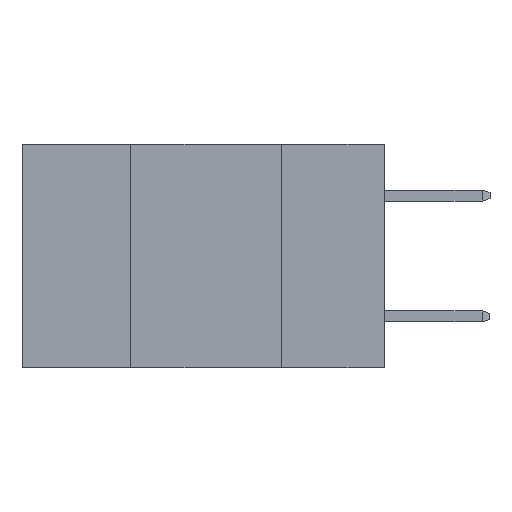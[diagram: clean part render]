
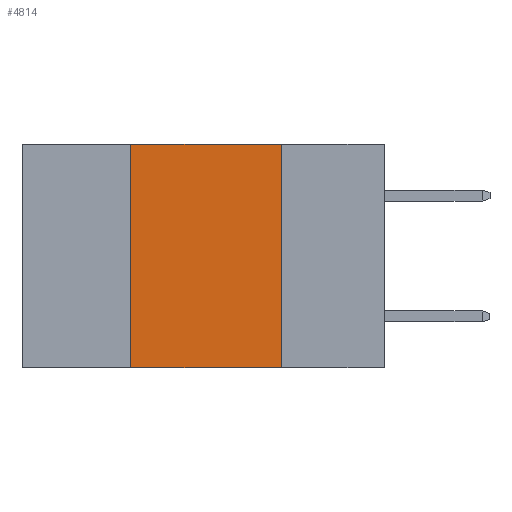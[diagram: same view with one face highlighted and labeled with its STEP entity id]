
A CAD part, left-side view. The second image highlights one B-rep face of the part: STEP entity #4814.
In plain terms, the highlighted planar face has unit normal (-1, 0, 0).
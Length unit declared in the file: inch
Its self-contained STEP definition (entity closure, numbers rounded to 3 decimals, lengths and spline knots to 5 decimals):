
#731 = EDGE_CURVE ( 'NONE', #6572, #828, #4768, .T. ) ;
#828 = VERTEX_POINT ( 'NONE', #8652 ) ;
#965 = DIRECTION ( 'NONE',  ( 0., 0., -1. ) ) ;
#1046 = CARTESIAN_POINT ( 'NONE',  ( 0., 0.17, 0. ) ) ;
#1332 = EDGE_CURVE ( 'NONE', #5861, #828, #8625, .T. ) ;
#1594 = CARTESIAN_POINT ( 'NONE',  ( 0., 0.42, -0.37 ) ) ;
#1639 = VECTOR ( 'NONE', #5365, 39.37008 ) ;
#2737 = FACE_OUTER_BOUND ( 'NONE', #8730, .T. ) ;
#4005 = CARTESIAN_POINT ( 'NONE',  ( 0., 0.6, -0.37 ) ) ;
#4096 = ORIENTED_EDGE ( 'NONE', *, *, #731, .T. ) ;
#4536 = VECTOR ( 'NONE', #7306, 39.37008 ) ;
#4649 = EDGE_CURVE ( 'NONE', #7013, #5861, #7054, .T. ) ;
#4768 = LINE ( 'NONE', #4005, #9449 ) ;
#4814 = ADVANCED_FACE ( 'NONE', ( #2737 ), #7819, .F. ) ;
#5096 = AXIS2_PLACEMENT_3D ( 'NONE', #7846, #7914, #7911 ) ;
#5365 = DIRECTION ( 'NONE',  ( 0., 0., 1. ) ) ;
#5779 = VECTOR ( 'NONE', #965, 39.37008 ) ;
#5861 = VERTEX_POINT ( 'NONE', #9203 ) ;
#6572 = VERTEX_POINT ( 'NONE', #1594 ) ;
#7013 = VERTEX_POINT ( 'NONE', #11663 ) ;
#7054 = LINE ( 'NONE', #11337, #4536 ) ;
#7306 = DIRECTION ( 'NONE',  ( 0., -1., 0. ) ) ;
#7819 = PLANE ( 'NONE',  #5096 ) ;
#7846 = CARTESIAN_POINT ( 'NONE',  ( 0., 0.6, 0. ) ) ;
#7911 = DIRECTION ( 'NONE',  ( 0., 0., -1. ) ) ;
#7914 = DIRECTION ( 'NONE',  ( 1., 0., 0. ) ) ;
#8625 = LINE ( 'NONE', #1046, #5779 ) ;
#8652 = CARTESIAN_POINT ( 'NONE',  ( 0., 0.17, -0.37 ) ) ;
#8730 = EDGE_LOOP ( 'NONE', ( #10747, #11785, #11339, #4096 ) ) ;
#8891 = EDGE_CURVE ( 'NONE', #6572, #7013, #11506, .T. ) ;
#9203 = CARTESIAN_POINT ( 'NONE',  ( 0., 0.17, 0. ) ) ;
#9244 = DIRECTION ( 'NONE',  ( 0., -1., 0. ) ) ;
#9449 = VECTOR ( 'NONE', #9244, 39.37008 ) ;
#9990 = CARTESIAN_POINT ( 'NONE',  ( 0., 0.42, 0. ) ) ;
#10747 = ORIENTED_EDGE ( 'NONE', *, *, #1332, .F. ) ;
#11337 = CARTESIAN_POINT ( 'NONE',  ( 0., 0.6, 0. ) ) ;
#11339 = ORIENTED_EDGE ( 'NONE', *, *, #8891, .F. ) ;
#11506 = LINE ( 'NONE', #9990, #1639 ) ;
#11663 = CARTESIAN_POINT ( 'NONE',  ( 0., 0.42, 0. ) ) ;
#11785 = ORIENTED_EDGE ( 'NONE', *, *, #4649, .F. ) ;
